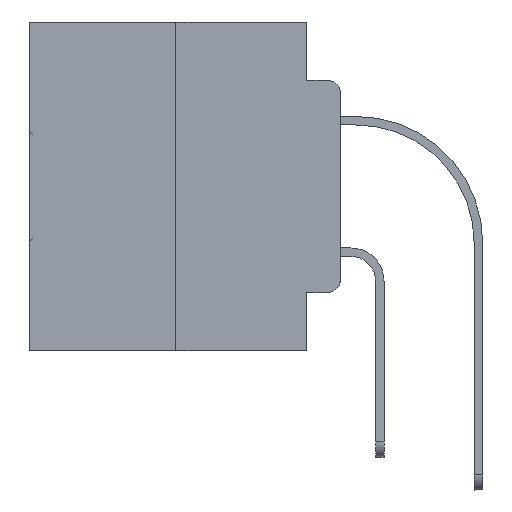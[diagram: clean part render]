
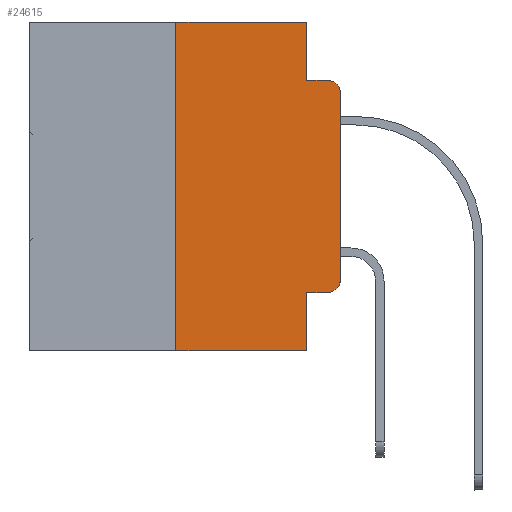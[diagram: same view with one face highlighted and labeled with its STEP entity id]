
A CAD part, left-side view. The second image highlights one B-rep face of the part: STEP entity #24615.
In plain terms, the highlighted planar face has unit normal (-1, 0, 0).
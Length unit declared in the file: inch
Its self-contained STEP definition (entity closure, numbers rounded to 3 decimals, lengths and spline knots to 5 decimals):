
#565 = DIRECTION ( 'NONE',  ( 0., 0., -1. ) ) ;
#1093 = ORIENTED_EDGE ( 'NONE', *, *, #22214, .T. ) ;
#1102 = DIRECTION ( 'NONE',  ( -1., 0., 0. ) ) ;
#1196 = CARTESIAN_POINT ( 'NONE',  ( 0., 0.473, 0. ) ) ;
#1554 = DIRECTION ( 'NONE',  ( 0., 0., -1. ) ) ;
#1625 = EDGE_CURVE ( 'NONE', #31788, #13678, #16514, .T. ) ;
#2479 = DIRECTION ( 'NONE',  ( 0., -1., 0. ) ) ;
#2492 = VECTOR ( 'NONE', #35042, 39.37008 ) ;
#2610 = CARTESIAN_POINT ( 'NONE',  ( 0., 0.051, -0.4115 ) ) ;
#2944 = DIRECTION ( 'NONE',  ( 0., 0., 1. ) ) ;
#4892 = EDGE_CURVE ( 'NONE', #32804, #32918, #27160, .T. ) ;
#5211 = CARTESIAN_POINT ( 'NONE',  ( 0., 0.051, -0.5 ) ) ;
#5362 = ORIENTED_EDGE ( 'NONE', *, *, #14255, .T. ) ;
#5444 = ORIENTED_EDGE ( 'NONE', *, *, #7834, .F. ) ;
#5675 = DIRECTION ( 'NONE',  ( 0., 0., -1. ) ) ;
#6235 = LINE ( 'NONE', #33816, #13742 ) ;
#6525 = VECTOR ( 'NONE', #9952, 39.37008 ) ;
#7155 = CARTESIAN_POINT ( 'NONE',  ( 0., 0.02, -0.4115 ) ) ;
#7273 = DIRECTION ( 'NONE',  ( 0., 0., -1. ) ) ;
#7528 = ORIENTED_EDGE ( 'NONE', *, *, #33280, .T. ) ;
#7834 = EDGE_CURVE ( 'NONE', #32804, #18550, #14626, .T. ) ;
#7861 = EDGE_CURVE ( 'NONE', #17253, #31788, #6235, .T. ) ;
#8143 = LINE ( 'NONE', #18253, #22567 ) ;
#9563 = CARTESIAN_POINT ( 'NONE',  ( 0., 0., -0.3915 ) ) ;
#9952 = DIRECTION ( 'NONE',  ( 0., -1., 0. ) ) ;
#10502 = CARTESIAN_POINT ( 'NONE',  ( 0., 0.02, -0.1085 ) ) ;
#12240 = AXIS2_PLACEMENT_3D ( 'NONE', #1196, #14623, #7273 ) ;
#12434 = CARTESIAN_POINT ( 'NONE',  ( 0., 0.051, 0. ) ) ;
#13355 = VERTEX_POINT ( 'NONE', #15152 ) ;
#13677 = EDGE_LOOP ( 'NONE', ( #7528, #5362, #33256, #22599, #14685, #13892, #1093, #5444, #26070, #30242 ) ) ;
#13678 = VERTEX_POINT ( 'NONE', #18458 ) ;
#13742 = VECTOR ( 'NONE', #20379, 39.37008 ) ;
#13892 = ORIENTED_EDGE ( 'NONE', *, *, #22986, .F. ) ;
#14255 = EDGE_CURVE ( 'NONE', #24039, #13355, #20998, .T. ) ;
#14623 = DIRECTION ( 'NONE',  ( 1., 0., 0. ) ) ;
#14626 = LINE ( 'NONE', #25582, #23509 ) ;
#14685 = ORIENTED_EDGE ( 'NONE', *, *, #7861, .F. ) ;
#15152 = CARTESIAN_POINT ( 'NONE',  ( 0., 0.02, -0.0885 ) ) ;
#15307 = VERTEX_POINT ( 'NONE', #18086 ) ;
#15356 = DIRECTION ( 'NONE',  ( 0., 0., 1. ) ) ;
#15452 = VECTOR ( 'NONE', #15356, 39.37008 ) ;
#15836 = CIRCLE ( 'NONE', #28444, 0.02 ) ;
#15902 = DIRECTION ( 'NONE',  ( 0., 0., -1. ) ) ;
#16244 = CARTESIAN_POINT ( 'NONE',  ( 0., 0.25, 0. ) ) ;
#16514 = LINE ( 'NONE', #27457, #24531 ) ;
#17253 = VERTEX_POINT ( 'NONE', #16244 ) ;
#18086 = CARTESIAN_POINT ( 'NONE',  ( 0., 0.25, -0.5 ) ) ;
#18253 = CARTESIAN_POINT ( 'NONE',  ( 0., 0.25, 0. ) ) ;
#18458 = CARTESIAN_POINT ( 'NONE',  ( 0., 0.051, -0.0885 ) ) ;
#18550 = VERTEX_POINT ( 'NONE', #5211 ) ;
#18607 = LINE ( 'NONE', #29559, #28089 ) ;
#20379 = DIRECTION ( 'NONE',  ( 0., -1., 0. ) ) ;
#20998 = CIRCLE ( 'NONE', #25044, 0.02 ) ;
#21468 = DIRECTION ( 'NONE',  ( -1., 0., 0. ) ) ;
#21770 = EDGE_CURVE ( 'NONE', #13678, #13355, #18607, .T. ) ;
#22214 = EDGE_CURVE ( 'NONE', #15307, #18550, #35401, .T. ) ;
#22567 = VECTOR ( 'NONE', #2944, 39.37008 ) ;
#22599 = ORIENTED_EDGE ( 'NONE', *, *, #1625, .F. ) ;
#22986 = EDGE_CURVE ( 'NONE', #15307, #17253, #8143, .T. ) ;
#23509 = VECTOR ( 'NONE', #1554, 39.37008 ) ;
#24039 = VERTEX_POINT ( 'NONE', #30117 ) ;
#24531 = VECTOR ( 'NONE', #565, 39.37008 ) ;
#24615 = ADVANCED_FACE ( 'NONE', ( #34511 ), #31299, .F. ) ;
#25044 = AXIS2_PLACEMENT_3D ( 'NONE', #10502, #1102, #15902 ) ;
#25582 = CARTESIAN_POINT ( 'NONE',  ( 0., 0.051, 0. ) ) ;
#26070 = ORIENTED_EDGE ( 'NONE', *, *, #4892, .T. ) ;
#26264 = VERTEX_POINT ( 'NONE', #9563 ) ;
#27160 = LINE ( 'NONE', #2610, #6525 ) ;
#27457 = CARTESIAN_POINT ( 'NONE',  ( 0., 0.051, 0. ) ) ;
#28089 = VECTOR ( 'NONE', #2479, 39.37008 ) ;
#28254 = EDGE_CURVE ( 'NONE', #32918, #26264, #15836, .T. ) ;
#28444 = AXIS2_PLACEMENT_3D ( 'NONE', #30235, #21468, #5675 ) ;
#29044 = CARTESIAN_POINT ( 'NONE',  ( 0., 0.051, -0.4115 ) ) ;
#29559 = CARTESIAN_POINT ( 'NONE',  ( 0., 0.051, -0.0885 ) ) ;
#30117 = CARTESIAN_POINT ( 'NONE',  ( 0., 0., -0.1085 ) ) ;
#30235 = CARTESIAN_POINT ( 'NONE',  ( 0., 0.02, -0.3915 ) ) ;
#30242 = ORIENTED_EDGE ( 'NONE', *, *, #28254, .T. ) ;
#31299 = PLANE ( 'NONE',  #12240 ) ;
#31673 = LINE ( 'NONE', #34706, #15452 ) ;
#31788 = VERTEX_POINT ( 'NONE', #12434 ) ;
#32718 = CARTESIAN_POINT ( 'NONE',  ( 0., 0.473, -0.5 ) ) ;
#32804 = VERTEX_POINT ( 'NONE', #29044 ) ;
#32918 = VERTEX_POINT ( 'NONE', #7155 ) ;
#33256 = ORIENTED_EDGE ( 'NONE', *, *, #21770, .F. ) ;
#33280 = EDGE_CURVE ( 'NONE', #26264, #24039, #31673, .T. ) ;
#33816 = CARTESIAN_POINT ( 'NONE',  ( 0., 0.473, 0. ) ) ;
#34511 = FACE_OUTER_BOUND ( 'NONE', #13677, .T. ) ;
#34706 = CARTESIAN_POINT ( 'NONE',  ( 0., 0., 0. ) ) ;
#35042 = DIRECTION ( 'NONE',  ( 0., -1., 0. ) ) ;
#35401 = LINE ( 'NONE', #32718, #2492 ) ;
